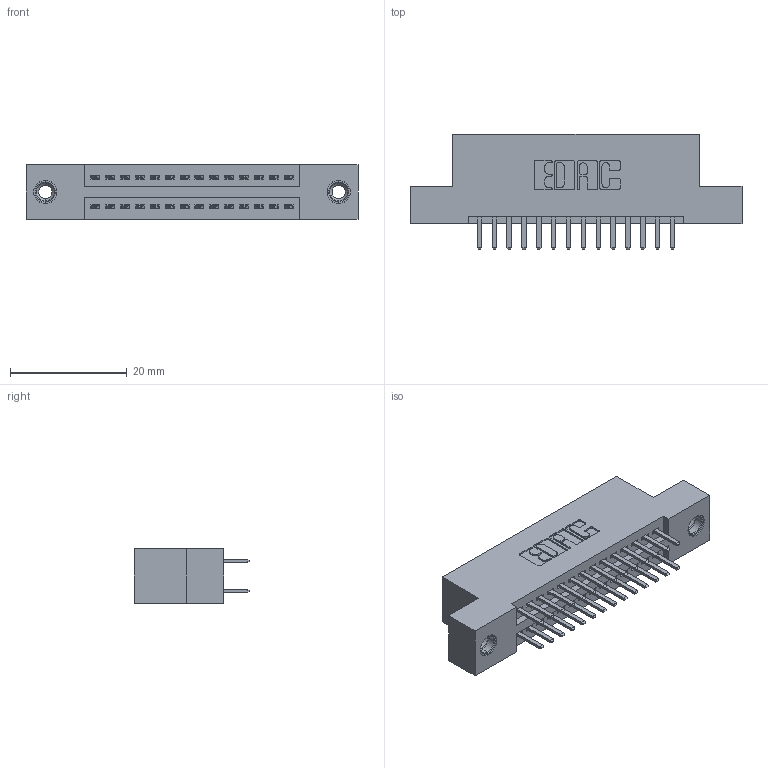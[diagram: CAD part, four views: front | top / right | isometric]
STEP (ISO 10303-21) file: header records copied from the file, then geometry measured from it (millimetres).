
FILE_DESCRIPTION (( 'STEP AP203' ), '1' );
FILE_NAME ('345-028-520-208.STEP', '2019-10-27T20:52:20', ( '' ), ( '' ), 'SwSTEP 2.0', 'SolidWorks 2016', '' );
FILE_SCHEMA (( 'CONFIG_CONTROL_DESIGN' ));
Length unit declared in the file: inch
Products named in the file (4): 345-028-520-208; 345-292-001_345-293-120; 345 Part_Flush Mounting Lugs - 0.156 Dia-TI; 345-250-001_345-250-003-102
Assembly tree (31 placements, depth 2):
  345-028-520-208
    345 Part_Flush Mounting Lugs - 0.156 Dia-TI
    345-292-001_345-293-120  x28
    345-250-001_345-250-003-102  x2
Bounding box: 56.77 x 19.68 x 9.4 mm (x, y, z)
Volume: 5235.9 mm3; surface area: 7184.4 mm2
Topology: 31 solids, 31 shells, 1698 faces, 4873 edges, 3166 vertices
Faces by surface type: plane 1092, cylinder 590, cone 12, torus 4
Entity records: 16054 total; most frequent: CARTESIAN_POINT 2711, ORIENTED_EDGE 2626, DIRECTION 2439, EDGE_CURVE 1313, VECTOR 1101, LINE 1101, VERTEX_POINT 868, AXIS2_PLACEMENT_3D 669
